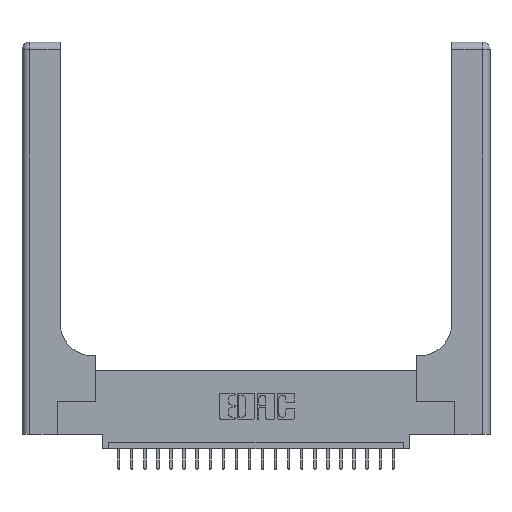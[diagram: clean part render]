
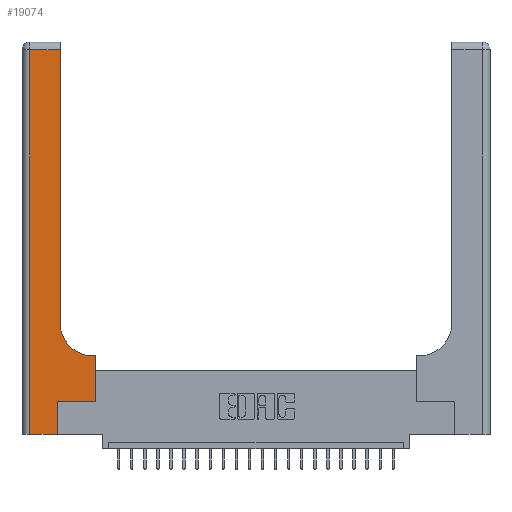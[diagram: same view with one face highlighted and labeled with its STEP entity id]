
A CAD part, top view. The second image highlights one B-rep face of the part: STEP entity #19074.
In plain terms, the highlighted planar face has unit normal (0, 0, 1).
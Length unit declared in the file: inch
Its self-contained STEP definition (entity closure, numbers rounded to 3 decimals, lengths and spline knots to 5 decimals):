
#42 = CARTESIAN_POINT ( 'NONE',  ( 0.2915, 2.94, 0.37 ) ) ;
#583 = ORIENTED_EDGE ( 'NONE', *, *, #11261, .T. ) ;
#626 = CARTESIAN_POINT ( 'NONE',  ( 0.5415, 0.6, 0.37 ) ) ;
#630 = EDGE_CURVE ( 'NONE', #22012, #11764, #7616, .T. ) ;
#1185 = VERTEX_POINT ( 'NONE', #20264 ) ;
#1543 = EDGE_CURVE ( 'NONE', #8966, #17751, #21885, .T. ) ;
#1618 = PLANE ( 'NONE',  #8027 ) ;
#2019 = ORIENTED_EDGE ( 'NONE', *, *, #23629, .T. ) ;
#2733 = EDGE_CURVE ( 'NONE', #4411, #22012, #9635, .T. ) ;
#2742 = ORIENTED_EDGE ( 'NONE', *, *, #630, .T. ) ;
#3588 = LINE ( 'NONE', #10599, #18222 ) ;
#4411 = VERTEX_POINT ( 'NONE', #15385 ) ;
#4933 = DIRECTION ( 'NONE',  ( 0., -1., 0. ) ) ;
#4972 = ORIENTED_EDGE ( 'NONE', *, *, #6745, .T. ) ;
#5213 = VECTOR ( 'NONE', #18788, 39.37008 ) ;
#5961 = CARTESIAN_POINT ( 'NONE',  ( 0.06, 0., 0.37 ) ) ;
#6550 = VERTEX_POINT ( 'NONE', #626 ) ;
#6745 = EDGE_CURVE ( 'NONE', #11764, #15890, #10892, .T. ) ;
#7045 = CARTESIAN_POINT ( 'NONE',  ( 0.269, 0.25, 0.37 ) ) ;
#7173 = CIRCLE ( 'NONE', #15954, 0.25 ) ;
#7226 = CARTESIAN_POINT ( 'NONE',  ( 0., 2.94, 0.37 ) ) ;
#7616 = LINE ( 'NONE', #7226, #5213 ) ;
#8027 = AXIS2_PLACEMENT_3D ( 'NONE', #9105, #20593, #11048 ) ;
#8080 = EDGE_CURVE ( 'NONE', #10588, #6550, #3588, .T. ) ;
#8389 = DIRECTION ( 'NONE',  ( 1., 0., 0. ) ) ;
#8966 = VERTEX_POINT ( 'NONE', #7045 ) ;
#9105 = CARTESIAN_POINT ( 'NONE',  ( 0., 3., 0.37 ) ) ;
#9635 = LINE ( 'NONE', #11572, #23930 ) ;
#10001 = CARTESIAN_POINT ( 'NONE',  ( 0.5585, 0.25, 0.37 ) ) ;
#10268 = DIRECTION ( 'NONE',  ( 1., 0., 0. ) ) ;
#10359 = FACE_OUTER_BOUND ( 'NONE', #16634, .T. ) ;
#10365 = LINE ( 'NONE', #19753, #19284 ) ;
#10588 = VERTEX_POINT ( 'NONE', #15502 ) ;
#10599 = CARTESIAN_POINT ( 'NONE',  ( 0.2915, 0.6, 0.37 ) ) ;
#10685 = DIRECTION ( 'NONE',  ( -1., 0., 0. ) ) ;
#10892 = LINE ( 'NONE', #20115, #24247 ) ;
#11048 = DIRECTION ( 'NONE',  ( -1., 0., 0. ) ) ;
#11255 = EDGE_CURVE ( 'NONE', #15890, #1185, #10365, .T. ) ;
#11261 = EDGE_CURVE ( 'NONE', #1185, #8966, #13661, .T. ) ;
#11513 = DIRECTION ( 'NONE',  ( 1., 0., 0. ) ) ;
#11572 = CARTESIAN_POINT ( 'NONE',  ( 0.2915, 3., 0.37 ) ) ;
#11764 = VERTEX_POINT ( 'NONE', #17204 ) ;
#12186 = DIRECTION ( 'NONE',  ( 0., 1., 0. ) ) ;
#12451 = ORIENTED_EDGE ( 'NONE', *, *, #20682, .T. ) ;
#12778 = DIRECTION ( 'NONE',  ( 0., 1., 0. ) ) ;
#13661 = LINE ( 'NONE', #23535, #15740 ) ;
#14409 = ORIENTED_EDGE ( 'NONE', *, *, #8080, .T. ) ;
#15175 = DIRECTION ( 'NONE',  ( 0., 0., -1. ) ) ;
#15385 = CARTESIAN_POINT ( 'NONE',  ( 0.2915, 0.85, 0.37 ) ) ;
#15502 = CARTESIAN_POINT ( 'NONE',  ( 0.5585, 0.6, 0.37 ) ) ;
#15740 = VECTOR ( 'NONE', #12186, 39.37008 ) ;
#15890 = VERTEX_POINT ( 'NONE', #5961 ) ;
#15954 = AXIS2_PLACEMENT_3D ( 'NONE', #22677, #15175, #11513 ) ;
#16634 = EDGE_LOOP ( 'NONE', ( #22229, #2742, #4972, #21646, #583, #18319, #12451, #14409, #2019 ) ) ;
#16875 = VECTOR ( 'NONE', #8389, 39.37008 ) ;
#17204 = CARTESIAN_POINT ( 'NONE',  ( 0.06, 2.94, 0.37 ) ) ;
#17751 = VERTEX_POINT ( 'NONE', #10001 ) ;
#18222 = VECTOR ( 'NONE', #10685, 39.37008 ) ;
#18319 = ORIENTED_EDGE ( 'NONE', *, *, #1543, .T. ) ;
#18651 = CARTESIAN_POINT ( 'NONE',  ( 0.5585, 0.25, 0.37 ) ) ;
#18788 = DIRECTION ( 'NONE',  ( -1., 0., 0. ) ) ;
#19074 = ADVANCED_FACE ( 'NONE', ( #10359 ), #1618, .F. ) ;
#19284 = VECTOR ( 'NONE', #10268, 39.37008 ) ;
#19496 = VECTOR ( 'NONE', #12778, 39.37008 ) ;
#19753 = CARTESIAN_POINT ( 'NONE',  ( 0., 0., 0.37 ) ) ;
#19810 = CARTESIAN_POINT ( 'NONE',  ( 0.269, 0.25, 0.37 ) ) ;
#20115 = CARTESIAN_POINT ( 'NONE',  ( 0.06, 3., 0.37 ) ) ;
#20264 = CARTESIAN_POINT ( 'NONE',  ( 0.269, 0., 0.37 ) ) ;
#20593 = DIRECTION ( 'NONE',  ( 0., 0., -1. ) ) ;
#20682 = EDGE_CURVE ( 'NONE', #17751, #10588, #22735, .T. ) ;
#21646 = ORIENTED_EDGE ( 'NONE', *, *, #11255, .T. ) ;
#21885 = LINE ( 'NONE', #19810, #16875 ) ;
#22012 = VERTEX_POINT ( 'NONE', #42 ) ;
#22229 = ORIENTED_EDGE ( 'NONE', *, *, #2733, .T. ) ;
#22677 = CARTESIAN_POINT ( 'NONE',  ( 0.5415, 0.85, 0.37 ) ) ;
#22735 = LINE ( 'NONE', #18651, #19496 ) ;
#22743 = DIRECTION ( 'NONE',  ( 0., 1., 0. ) ) ;
#23535 = CARTESIAN_POINT ( 'NONE',  ( 0.269, 0., 0.37 ) ) ;
#23629 = EDGE_CURVE ( 'NONE', #6550, #4411, #7173, .T. ) ;
#23930 = VECTOR ( 'NONE', #22743, 39.37008 ) ;
#24247 = VECTOR ( 'NONE', #4933, 39.37008 ) ;
